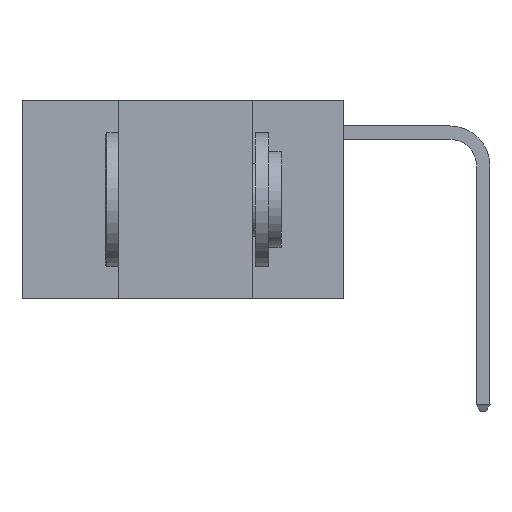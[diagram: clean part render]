
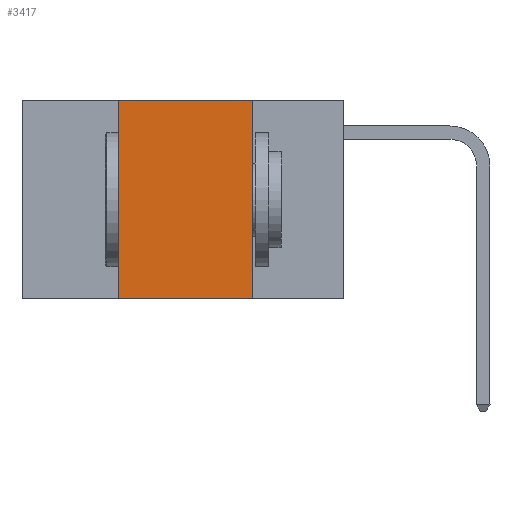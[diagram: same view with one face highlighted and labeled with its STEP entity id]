
A CAD part, left-side view. The second image highlights one B-rep face of the part: STEP entity #3417.
In plain terms, the highlighted planar face has unit normal (-1, 0, 0).
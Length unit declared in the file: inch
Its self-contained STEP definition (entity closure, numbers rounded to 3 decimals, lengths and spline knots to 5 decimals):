
#885 = VERTEX_POINT ( 'NONE', #15469 ) ;
#1212 = EDGE_CURVE ( 'NONE', #5244, #9833, #16846, .T. ) ;
#1492 = DIRECTION ( 'NONE',  ( 0., -1., 0. ) ) ;
#1514 = CARTESIAN_POINT ( 'NONE',  ( 0., 0.6, 0. ) ) ;
#1733 = FACE_OUTER_BOUND ( 'NONE', #18735, .T. ) ;
#2974 = VECTOR ( 'NONE', #8851, 39.37008 ) ;
#3071 = DIRECTION ( 'NONE',  ( 0., 0., -1. ) ) ;
#3191 = CARTESIAN_POINT ( 'NONE',  ( 0., 0.6, 0. ) ) ;
#3417 = ADVANCED_FACE ( 'NONE', ( #1733 ), #6696, .F. ) ;
#4326 = EDGE_CURVE ( 'NONE', #14194, #9833, #17069, .T. ) ;
#5244 = VERTEX_POINT ( 'NONE', #18484 ) ;
#5535 = ORIENTED_EDGE ( 'NONE', *, *, #9477, .F. ) ;
#6191 = ORIENTED_EDGE ( 'NONE', *, *, #4326, .T. ) ;
#6540 = VECTOR ( 'NONE', #21884, 39.37008 ) ;
#6696 = PLANE ( 'NONE',  #17556 ) ;
#8387 = CARTESIAN_POINT ( 'NONE',  ( 0., 0.42, -0.37 ) ) ;
#8624 = DIRECTION ( 'NONE',  ( 1., 0., 0. ) ) ;
#8800 = EDGE_CURVE ( 'NONE', #885, #5244, #13445, .T. ) ;
#8851 = DIRECTION ( 'NONE',  ( 0., 0., 1. ) ) ;
#9477 = EDGE_CURVE ( 'NONE', #14194, #885, #13983, .T. ) ;
#9833 = VERTEX_POINT ( 'NONE', #18752 ) ;
#11627 = ORIENTED_EDGE ( 'NONE', *, *, #1212, .F. ) ;
#13445 = LINE ( 'NONE', #3191, #6540 ) ;
#13983 = LINE ( 'NONE', #14339, #2974 ) ;
#14194 = VERTEX_POINT ( 'NONE', #8387 ) ;
#14339 = CARTESIAN_POINT ( 'NONE',  ( 0., 0.42, 0. ) ) ;
#15469 = CARTESIAN_POINT ( 'NONE',  ( 0., 0.42, 0. ) ) ;
#16846 = LINE ( 'NONE', #19180, #22460 ) ;
#17069 = LINE ( 'NONE', #17299, #21194 ) ;
#17299 = CARTESIAN_POINT ( 'NONE',  ( 0., 0.6, -0.37 ) ) ;
#17556 = AXIS2_PLACEMENT_3D ( 'NONE', #1514, #8624, #22338 ) ;
#18484 = CARTESIAN_POINT ( 'NONE',  ( 0., 0.17, 0. ) ) ;
#18735 = EDGE_LOOP ( 'NONE', ( #11627, #19011, #5535, #6191 ) ) ;
#18752 = CARTESIAN_POINT ( 'NONE',  ( 0., 0.17, -0.37 ) ) ;
#19011 = ORIENTED_EDGE ( 'NONE', *, *, #8800, .F. ) ;
#19180 = CARTESIAN_POINT ( 'NONE',  ( 0., 0.17, 0. ) ) ;
#21194 = VECTOR ( 'NONE', #1492, 39.37008 ) ;
#21884 = DIRECTION ( 'NONE',  ( 0., -1., 0. ) ) ;
#22338 = DIRECTION ( 'NONE',  ( 0., 0., -1. ) ) ;
#22460 = VECTOR ( 'NONE', #3071, 39.37008 ) ;
